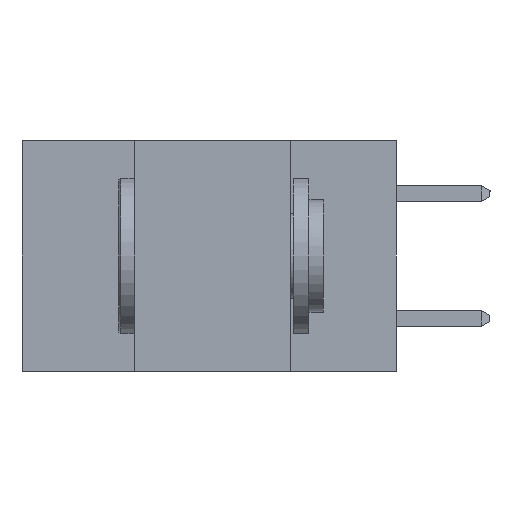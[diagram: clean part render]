
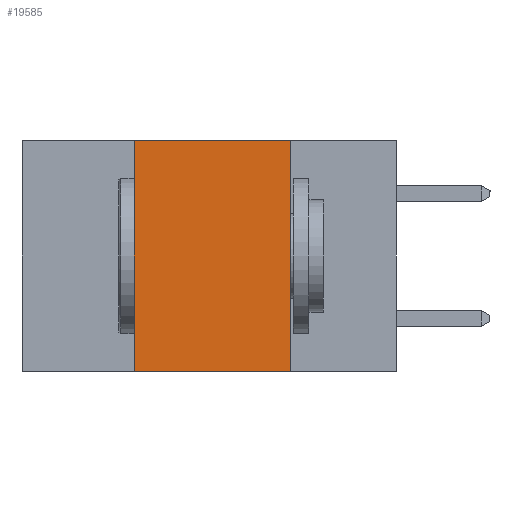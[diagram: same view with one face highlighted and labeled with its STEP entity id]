
A CAD part, left-side view. The second image highlights one B-rep face of the part: STEP entity #19585.
In plain terms, the highlighted planar face has unit normal (-1, 0, 0).
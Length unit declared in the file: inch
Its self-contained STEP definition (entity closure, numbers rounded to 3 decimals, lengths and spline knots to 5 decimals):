
#401 = DIRECTION ( 'NONE',  ( 0., -1., 0. ) ) ;
#1086 = EDGE_CURVE ( 'NONE', #9518, #19481, #10300, .T. ) ;
#1553 = VECTOR ( 'NONE', #2946, 39.37008 ) ;
#1949 = FACE_OUTER_BOUND ( 'NONE', #16087, .T. ) ;
#2946 = DIRECTION ( 'NONE',  ( 0., 0., -1. ) ) ;
#4298 = DIRECTION ( 'NONE',  ( 0., 0., -1. ) ) ;
#4462 = EDGE_CURVE ( 'NONE', #10865, #16563, #6759, .T. ) ;
#5159 = ORIENTED_EDGE ( 'NONE', *, *, #1086, .T. ) ;
#6416 = VECTOR ( 'NONE', #7958, 39.37008 ) ;
#6759 = LINE ( 'NONE', #10921, #25200 ) ;
#7958 = DIRECTION ( 'NONE',  ( 0., -1., 0. ) ) ;
#8449 = DIRECTION ( 'NONE',  ( 1., 0., 0. ) ) ;
#9142 = ORIENTED_EDGE ( 'NONE', *, *, #20633, .F. ) ;
#9442 = CARTESIAN_POINT ( 'NONE',  ( 0., 0.17, -0.37 ) ) ;
#9518 = VERTEX_POINT ( 'NONE', #15531 ) ;
#10300 = LINE ( 'NONE', #12236, #6416 ) ;
#10628 = ORIENTED_EDGE ( 'NONE', *, *, #14725, .F. ) ;
#10865 = VERTEX_POINT ( 'NONE', #26592 ) ;
#10921 = CARTESIAN_POINT ( 'NONE',  ( 0., 0.6, 0. ) ) ;
#12215 = VECTOR ( 'NONE', #12288, 39.37008 ) ;
#12236 = CARTESIAN_POINT ( 'NONE',  ( 0., 0.6, -0.37 ) ) ;
#12288 = DIRECTION ( 'NONE',  ( 0., 0., 1. ) ) ;
#12417 = LINE ( 'NONE', #21009, #12215 ) ;
#13318 = LINE ( 'NONE', #9442, #1553 ) ;
#14197 = CARTESIAN_POINT ( 'NONE',  ( 0., 0.17, 0. ) ) ;
#14725 = EDGE_CURVE ( 'NONE', #9518, #10865, #12417, .T. ) ;
#14821 = CARTESIAN_POINT ( 'NONE',  ( 0., 0.6, 0. ) ) ;
#15531 = CARTESIAN_POINT ( 'NONE',  ( 0., 0.42, -0.37 ) ) ;
#16086 = ORIENTED_EDGE ( 'NONE', *, *, #4462, .F. ) ;
#16087 = EDGE_LOOP ( 'NONE', ( #9142, #16086, #10628, #5159 ) ) ;
#16096 = AXIS2_PLACEMENT_3D ( 'NONE', #14821, #8449, #4298 ) ;
#16563 = VERTEX_POINT ( 'NONE', #14197 ) ;
#19481 = VERTEX_POINT ( 'NONE', #27014 ) ;
#19585 = ADVANCED_FACE ( 'NONE', ( #1949 ), #20778, .F. ) ;
#20633 = EDGE_CURVE ( 'NONE', #16563, #19481, #13318, .T. ) ;
#20778 = PLANE ( 'NONE',  #16096 ) ;
#21009 = CARTESIAN_POINT ( 'NONE',  ( 0., 0.42, -0.37 ) ) ;
#25200 = VECTOR ( 'NONE', #401, 39.37008 ) ;
#26592 = CARTESIAN_POINT ( 'NONE',  ( 0., 0.42, 0. ) ) ;
#27014 = CARTESIAN_POINT ( 'NONE',  ( 0., 0.17, -0.37 ) ) ;
